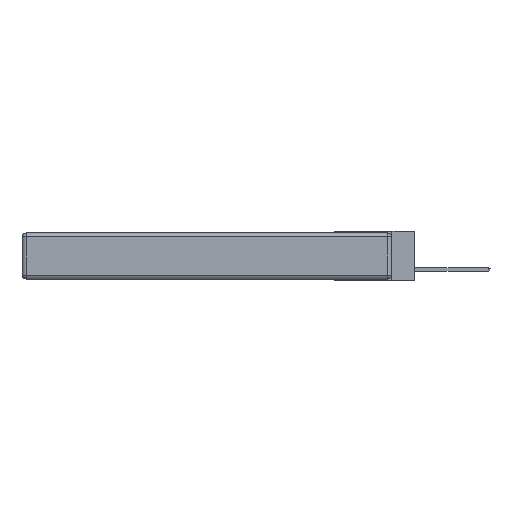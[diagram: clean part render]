
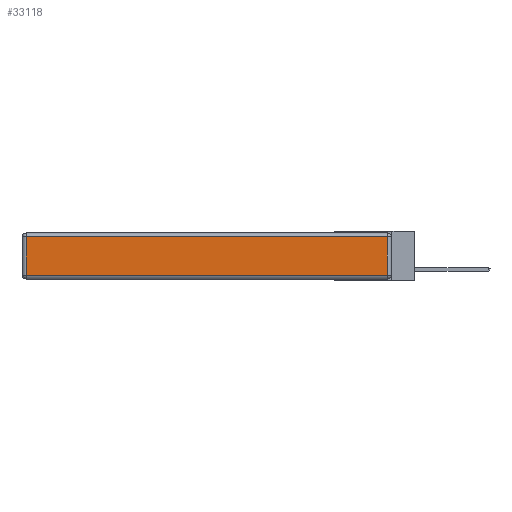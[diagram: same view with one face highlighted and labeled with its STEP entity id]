
A CAD part, left-side view. The second image highlights one B-rep face of the part: STEP entity #33118.
In plain terms, the highlighted planar face has unit normal (-1, 0, 0).
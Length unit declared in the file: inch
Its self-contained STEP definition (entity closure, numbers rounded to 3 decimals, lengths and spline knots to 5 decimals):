
#710 = VERTEX_POINT ( 'NONE', #4494 ) ;
#771 = ORIENTED_EDGE ( 'NONE', *, *, #20081, .T. ) ;
#846 = VERTEX_POINT ( 'NONE', #33330 ) ;
#939 = DIRECTION ( 'NONE',  ( 0., 0., 1. ) ) ;
#2006 = VECTOR ( 'NONE', #14924, 39.37008 ) ;
#2040 = EDGE_LOOP ( 'NONE', ( #771, #13234, #11616, #6880 ) ) ;
#3937 = DIRECTION ( 'NONE',  ( -1., 0., 0. ) ) ;
#4494 = CARTESIAN_POINT ( 'NONE',  ( 0., 2.72, -0.313 ) ) ;
#5427 = DIRECTION ( 'NONE',  ( 0., -1., 0. ) ) ;
#6880 = ORIENTED_EDGE ( 'NONE', *, *, #33508, .T. ) ;
#9250 = PLANE ( 'NONE',  #9788 ) ;
#9788 = AXIS2_PLACEMENT_3D ( 'NONE', #11597, #3937, #939 ) ;
#11597 = CARTESIAN_POINT ( 'NONE',  ( 0., 0., -0.343 ) ) ;
#11616 = ORIENTED_EDGE ( 'NONE', *, *, #21546, .T. ) ;
#13234 = ORIENTED_EDGE ( 'NONE', *, *, #15604, .T. ) ;
#14924 = DIRECTION ( 'NONE',  ( 0., 1., 0. ) ) ;
#15604 = EDGE_CURVE ( 'NONE', #846, #20032, #28500, .T. ) ;
#17589 = LINE ( 'NONE', #20206, #25439 ) ;
#18292 = LINE ( 'NONE', #18465, #19529 ) ;
#18465 = CARTESIAN_POINT ( 'NONE',  ( 0., 0., -0.313 ) ) ;
#19321 = LINE ( 'NONE', #20108, #2006 ) ;
#19529 = VECTOR ( 'NONE', #5427, 39.37008 ) ;
#20032 = VERTEX_POINT ( 'NONE', #34113 ) ;
#20081 = EDGE_CURVE ( 'NONE', #710, #846, #18292, .T. ) ;
#20108 = CARTESIAN_POINT ( 'NONE',  ( 0., 2.75, -0.03 ) ) ;
#20206 = CARTESIAN_POINT ( 'NONE',  ( 0., 2.72, -0.343 ) ) ;
#20650 = CARTESIAN_POINT ( 'NONE',  ( 0., 0.03, -0.343 ) ) ;
#21546 = EDGE_CURVE ( 'NONE', #20032, #31709, #19321, .T. ) ;
#23357 = FACE_OUTER_BOUND ( 'NONE', #2040, .T. ) ;
#25439 = VECTOR ( 'NONE', #25747, 39.37008 ) ;
#25747 = DIRECTION ( 'NONE',  ( 0., 0., -1. ) ) ;
#28460 = DIRECTION ( 'NONE',  ( 0., 0., 1. ) ) ;
#28500 = LINE ( 'NONE', #20650, #30545 ) ;
#30545 = VECTOR ( 'NONE', #28460, 39.37008 ) ;
#31709 = VERTEX_POINT ( 'NONE', #32580 ) ;
#32580 = CARTESIAN_POINT ( 'NONE',  ( 0., 2.72, -0.03 ) ) ;
#33118 = ADVANCED_FACE ( 'NONE', ( #23357 ), #9250, .T. ) ;
#33330 = CARTESIAN_POINT ( 'NONE',  ( 0., 0.03, -0.313 ) ) ;
#33508 = EDGE_CURVE ( 'NONE', #31709, #710, #17589, .T. ) ;
#34113 = CARTESIAN_POINT ( 'NONE',  ( 0., 0.03, -0.03 ) ) ;
